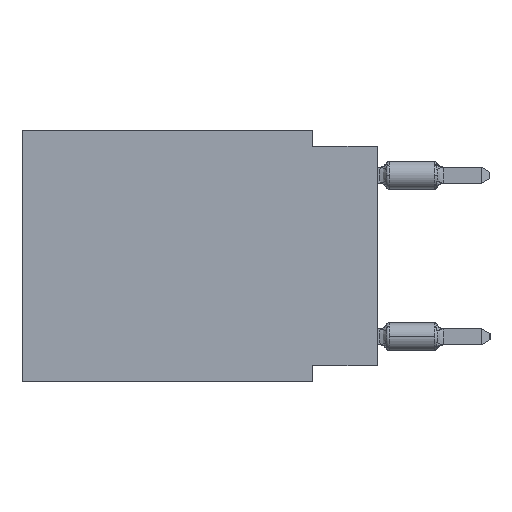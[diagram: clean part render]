
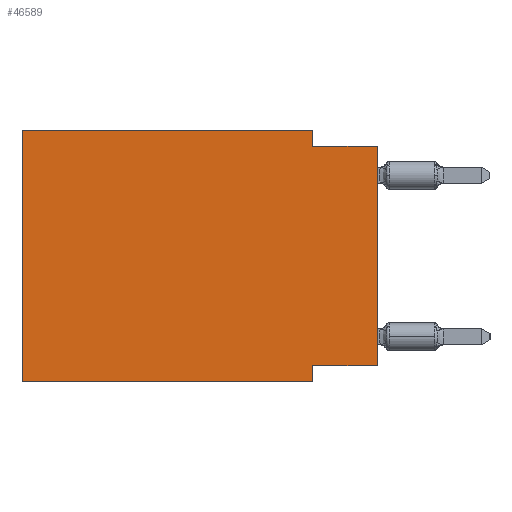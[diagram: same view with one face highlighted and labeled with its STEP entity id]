
A CAD part, left-side view. The second image highlights one B-rep face of the part: STEP entity #46589.
In plain terms, the highlighted planar face has unit normal (-1, 0, 0).
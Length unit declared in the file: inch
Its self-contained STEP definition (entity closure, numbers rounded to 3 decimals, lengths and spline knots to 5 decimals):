
#946 = VECTOR ( 'NONE', #29922, 39.37008 ) ;
#1921 = EDGE_CURVE ( 'NONE', #35161, #4580, #41297, .T. ) ;
#2175 = LINE ( 'NONE', #16522, #41287 ) ;
#2248 = VECTOR ( 'NONE', #8259, 39.37008 ) ;
#2394 = CARTESIAN_POINT ( 'NONE',  ( 0., 0.1, -0.365 ) ) ;
#2991 = ORIENTED_EDGE ( 'NONE', *, *, #16510, .F. ) ;
#3547 = VECTOR ( 'NONE', #24541, 39.37008 ) ;
#3802 = CARTESIAN_POINT ( 'NONE',  ( 0., 0.1, 0. ) ) ;
#3915 = CARTESIAN_POINT ( 'NONE',  ( 0., 0.1, -0.025 ) ) ;
#4580 = VERTEX_POINT ( 'NONE', #10759 ) ;
#4764 = EDGE_CURVE ( 'NONE', #35161, #23991, #39984, .T. ) ;
#5128 = AXIS2_PLACEMENT_3D ( 'NONE', #14037, #6501, #42345 ) ;
#6501 = DIRECTION ( 'NONE',  ( 1., 0., 0. ) ) ;
#8211 = EDGE_CURVE ( 'NONE', #12146, #35984, #2175, .T. ) ;
#8259 = DIRECTION ( 'NONE',  ( 0., 1., 0. ) ) ;
#9513 = ORIENTED_EDGE ( 'NONE', *, *, #4764, .F. ) ;
#10269 = PLANE ( 'NONE',  #5128 ) ;
#10759 = CARTESIAN_POINT ( 'NONE',  ( 0., 0.1, -0.39 ) ) ;
#11320 = VECTOR ( 'NONE', #41062, 39.37008 ) ;
#11829 = EDGE_CURVE ( 'NONE', #13350, #4580, #32544, .T. ) ;
#12146 = VERTEX_POINT ( 'NONE', #37503 ) ;
#13350 = VERTEX_POINT ( 'NONE', #2394 ) ;
#13573 = FACE_OUTER_BOUND ( 'NONE', #20135, .T. ) ;
#14023 = ORIENTED_EDGE ( 'NONE', *, *, #8211, .T. ) ;
#14037 = CARTESIAN_POINT ( 'NONE',  ( 0., 0.55, 0. ) ) ;
#14696 = ORIENTED_EDGE ( 'NONE', *, *, #1921, .T. ) ;
#14855 = EDGE_CURVE ( 'NONE', #12146, #13350, #43863, .T. ) ;
#15319 = CARTESIAN_POINT ( 'NONE',  ( 0., 0., -0.365 ) ) ;
#15731 = VERTEX_POINT ( 'NONE', #3915 ) ;
#16510 = EDGE_CURVE ( 'NONE', #15731, #35984, #35250, .T. ) ;
#16522 = CARTESIAN_POINT ( 'NONE',  ( 0., 0., 0. ) ) ;
#18941 = CARTESIAN_POINT ( 'NONE',  ( 0., 0., -0.025 ) ) ;
#20135 = EDGE_LOOP ( 'NONE', ( #14023, #2991, #20910, #23602, #9513, #14696, #23100, #25596 ) ) ;
#20439 = EDGE_CURVE ( 'NONE', #25605, #15731, #28995, .T. ) ;
#20893 = CARTESIAN_POINT ( 'NONE',  ( 0., 0.55, 0. ) ) ;
#20910 = ORIENTED_EDGE ( 'NONE', *, *, #20439, .F. ) ;
#21089 = DIRECTION ( 'NONE',  ( 0., -1., 0. ) ) ;
#21591 = DIRECTION ( 'NONE',  ( 0., -1., 0. ) ) ;
#21795 = DIRECTION ( 'NONE',  ( 0., 0., 1. ) ) ;
#22345 = EDGE_CURVE ( 'NONE', #23991, #25605, #38848, .T. ) ;
#23100 = ORIENTED_EDGE ( 'NONE', *, *, #11829, .F. ) ;
#23344 = CARTESIAN_POINT ( 'NONE',  ( 0., 0.55, -0.39 ) ) ;
#23602 = ORIENTED_EDGE ( 'NONE', *, *, #22345, .F. ) ;
#23991 = VERTEX_POINT ( 'NONE', #29250 ) ;
#24310 = CARTESIAN_POINT ( 'NONE',  ( 0., 0.1, -0.39 ) ) ;
#24541 = DIRECTION ( 'NONE',  ( 0., 0., -1. ) ) ;
#25596 = ORIENTED_EDGE ( 'NONE', *, *, #14855, .F. ) ;
#25605 = VERTEX_POINT ( 'NONE', #3802 ) ;
#28163 = VECTOR ( 'NONE', #21591, 39.37008 ) ;
#28995 = LINE ( 'NONE', #43416, #946 ) ;
#29250 = CARTESIAN_POINT ( 'NONE',  ( 0., 0.55, 0. ) ) ;
#29922 = DIRECTION ( 'NONE',  ( 0., 0., -1. ) ) ;
#31052 = VECTOR ( 'NONE', #21795, 39.37008 ) ;
#32544 = LINE ( 'NONE', #24310, #3547 ) ;
#34428 = DIRECTION ( 'NONE',  ( 0., 0., 1. ) ) ;
#35161 = VERTEX_POINT ( 'NONE', #44858 ) ;
#35250 = LINE ( 'NONE', #35722, #45976 ) ;
#35722 = CARTESIAN_POINT ( 'NONE',  ( 0., 0., -0.025 ) ) ;
#35984 = VERTEX_POINT ( 'NONE', #18941 ) ;
#37503 = CARTESIAN_POINT ( 'NONE',  ( 0., 0., -0.365 ) ) ;
#38848 = LINE ( 'NONE', #20893, #28163 ) ;
#39984 = LINE ( 'NONE', #43515, #31052 ) ;
#41062 = DIRECTION ( 'NONE',  ( 0., -1., 0. ) ) ;
#41287 = VECTOR ( 'NONE', #34428, 39.37008 ) ;
#41297 = LINE ( 'NONE', #23344, #11320 ) ;
#42345 = DIRECTION ( 'NONE',  ( 0., 0., -1. ) ) ;
#43416 = CARTESIAN_POINT ( 'NONE',  ( 0., 0.1, 0. ) ) ;
#43515 = CARTESIAN_POINT ( 'NONE',  ( 0., 0.55, 0. ) ) ;
#43863 = LINE ( 'NONE', #15319, #2248 ) ;
#44858 = CARTESIAN_POINT ( 'NONE',  ( 0., 0.55, -0.39 ) ) ;
#45976 = VECTOR ( 'NONE', #21089, 39.37008 ) ;
#46589 = ADVANCED_FACE ( 'NONE', ( #13573 ), #10269, .F. ) ;
